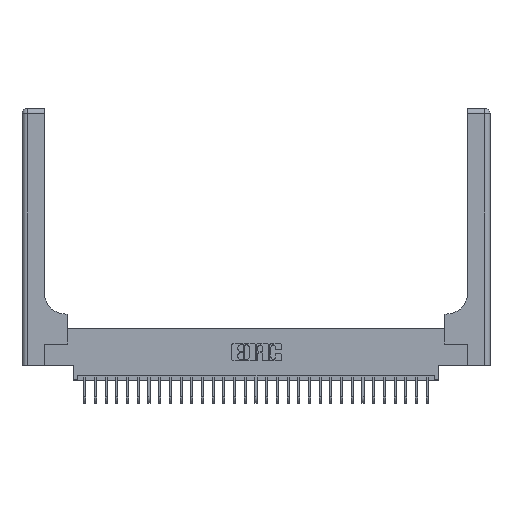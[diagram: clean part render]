
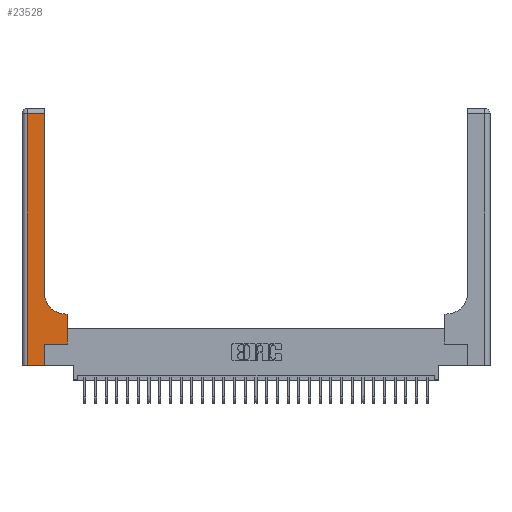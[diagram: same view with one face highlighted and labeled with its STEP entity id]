
A CAD part, top view. The second image highlights one B-rep face of the part: STEP entity #23528.
In plain terms, the highlighted planar face has unit normal (0, 0, 1).
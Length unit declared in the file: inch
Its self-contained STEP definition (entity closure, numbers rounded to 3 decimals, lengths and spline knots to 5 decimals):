
#187 = CIRCLE ( 'NONE', #4634, 0.25 ) ;
#490 = VERTEX_POINT ( 'NONE', #6327 ) ;
#572 = LINE ( 'NONE', #4886, #12703 ) ;
#697 = EDGE_CURVE ( 'NONE', #6568, #25458, #572, .T. ) ;
#1057 = DIRECTION ( 'NONE',  ( -1., 0., 0. ) ) ;
#1361 = EDGE_CURVE ( 'NONE', #18447, #6568, #9116, .T. ) ;
#1931 = DIRECTION ( 'NONE',  ( -1., 0., 0. ) ) ;
#1998 = ORIENTED_EDGE ( 'NONE', *, *, #1361, .T. ) ;
#2088 = VERTEX_POINT ( 'NONE', #10084 ) ;
#2521 = LINE ( 'NONE', #21611, #16424 ) ;
#2609 = EDGE_CURVE ( 'NONE', #25458, #490, #5243, .T. ) ;
#2795 = VERTEX_POINT ( 'NONE', #27377 ) ;
#3285 = CARTESIAN_POINT ( 'NONE',  ( 0., 3., 0.37 ) ) ;
#3723 = EDGE_LOOP ( 'NONE', ( #6628, #15226, #1998, #6989, #12238, #17588, #5731, #19811, #22344 ) ) ;
#4164 = VERTEX_POINT ( 'NONE', #24253 ) ;
#4634 = AXIS2_PLACEMENT_3D ( 'NONE', #5644, #14101, #20231 ) ;
#4886 = CARTESIAN_POINT ( 'NONE',  ( 0., 0., 0.37 ) ) ;
#5104 = FACE_OUTER_BOUND ( 'NONE', #3723, .T. ) ;
#5240 = PLANE ( 'NONE',  #25297 ) ;
#5243 = LINE ( 'NONE', #26823, #17836 ) ;
#5357 = EDGE_CURVE ( 'NONE', #9269, #2088, #5369, .T. ) ;
#5369 = LINE ( 'NONE', #26806, #14291 ) ;
#5548 = EDGE_CURVE ( 'NONE', #4164, #2795, #15659, .T. ) ;
#5557 = VERTEX_POINT ( 'NONE', #23989 ) ;
#5637 = LINE ( 'NONE', #27065, #22679 ) ;
#5644 = CARTESIAN_POINT ( 'NONE',  ( 0.51, 0.85, 0.37 ) ) ;
#5685 = CARTESIAN_POINT ( 'NONE',  ( 0.06, 0., 0.37 ) ) ;
#5731 = ORIENTED_EDGE ( 'NONE', *, *, #9908, .T. ) ;
#6327 = CARTESIAN_POINT ( 'NONE',  ( 0.265, 0.25, 0.37 ) ) ;
#6412 = CARTESIAN_POINT ( 'NONE',  ( 0.528, 0.6, 0.37 ) ) ;
#6568 = VERTEX_POINT ( 'NONE', #5685 ) ;
#6628 = ORIENTED_EDGE ( 'NONE', *, *, #5548, .T. ) ;
#6989 = ORIENTED_EDGE ( 'NONE', *, *, #697, .T. ) ;
#7081 = DIRECTION ( 'NONE',  ( 0., 0., -1. ) ) ;
#9116 = LINE ( 'NONE', #15515, #19836 ) ;
#9201 = EDGE_CURVE ( 'NONE', #2795, #18447, #19308, .T. ) ;
#9269 = VERTEX_POINT ( 'NONE', #6412 ) ;
#9908 = EDGE_CURVE ( 'NONE', #5557, #9269, #5637, .T. ) ;
#10084 = CARTESIAN_POINT ( 'NONE',  ( 0.51, 0.6, 0.37 ) ) ;
#10893 = DIRECTION ( 'NONE',  ( 1., 0., 0. ) ) ;
#11461 = DIRECTION ( 'NONE',  ( 0., -1., 0. ) ) ;
#12238 = ORIENTED_EDGE ( 'NONE', *, *, #2609, .T. ) ;
#12703 = VECTOR ( 'NONE', #24099, 39.37008 ) ;
#12767 = CARTESIAN_POINT ( 'NONE',  ( 0., 2.94, 0.37 ) ) ;
#13825 = DIRECTION ( 'NONE',  ( 0., 1., 0. ) ) ;
#14101 = DIRECTION ( 'NONE',  ( 0., 0., -1. ) ) ;
#14291 = VECTOR ( 'NONE', #18147, 39.37008 ) ;
#15226 = ORIENTED_EDGE ( 'NONE', *, *, #9201, .T. ) ;
#15373 = CARTESIAN_POINT ( 'NONE',  ( 0.26, 3., 0.37 ) ) ;
#15402 = EDGE_CURVE ( 'NONE', #2088, #4164, #187, .T. ) ;
#15515 = CARTESIAN_POINT ( 'NONE',  ( 0.06, 3., 0.37 ) ) ;
#15659 = LINE ( 'NONE', #15373, #20514 ) ;
#16055 = VECTOR ( 'NONE', #1931, 39.37008 ) ;
#16424 = VECTOR ( 'NONE', #10893, 39.37008 ) ;
#17588 = ORIENTED_EDGE ( 'NONE', *, *, #17788, .T. ) ;
#17788 = EDGE_CURVE ( 'NONE', #490, #5557, #2521, .T. ) ;
#17836 = VECTOR ( 'NONE', #26676, 39.37008 ) ;
#18147 = DIRECTION ( 'NONE',  ( -1., 0., 0. ) ) ;
#18447 = VERTEX_POINT ( 'NONE', #23054 ) ;
#19308 = LINE ( 'NONE', #12767, #16055 ) ;
#19811 = ORIENTED_EDGE ( 'NONE', *, *, #5357, .T. ) ;
#19836 = VECTOR ( 'NONE', #11461, 39.37008 ) ;
#20231 = DIRECTION ( 'NONE',  ( 1., 0., 0. ) ) ;
#20514 = VECTOR ( 'NONE', #23844, 39.37008 ) ;
#21611 = CARTESIAN_POINT ( 'NONE',  ( 0.265, 0.25, 0.37 ) ) ;
#22162 = CARTESIAN_POINT ( 'NONE',  ( 0.265, 0., 0.37 ) ) ;
#22344 = ORIENTED_EDGE ( 'NONE', *, *, #15402, .T. ) ;
#22679 = VECTOR ( 'NONE', #13825, 39.37008 ) ;
#23054 = CARTESIAN_POINT ( 'NONE',  ( 0.06, 2.94, 0.37 ) ) ;
#23528 = ADVANCED_FACE ( 'NONE', ( #5104 ), #5240, .F. ) ;
#23844 = DIRECTION ( 'NONE',  ( 0., 1., 0. ) ) ;
#23989 = CARTESIAN_POINT ( 'NONE',  ( 0.528, 0.25, 0.37 ) ) ;
#24099 = DIRECTION ( 'NONE',  ( 1., 0., 0. ) ) ;
#24253 = CARTESIAN_POINT ( 'NONE',  ( 0.26, 0.85, 0.37 ) ) ;
#25297 = AXIS2_PLACEMENT_3D ( 'NONE', #3285, #7081, #1057 ) ;
#25458 = VERTEX_POINT ( 'NONE', #22162 ) ;
#26676 = DIRECTION ( 'NONE',  ( 0., 1., 0. ) ) ;
#26806 = CARTESIAN_POINT ( 'NONE',  ( 0.26, 0.6, 0.37 ) ) ;
#26823 = CARTESIAN_POINT ( 'NONE',  ( 0.265, 0., 0.37 ) ) ;
#27065 = CARTESIAN_POINT ( 'NONE',  ( 0.528, 0.25, 0.37 ) ) ;
#27377 = CARTESIAN_POINT ( 'NONE',  ( 0.26, 2.94, 0.37 ) ) ;
